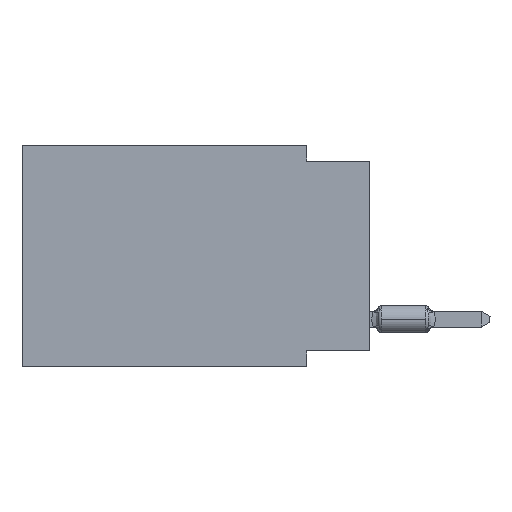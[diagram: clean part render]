
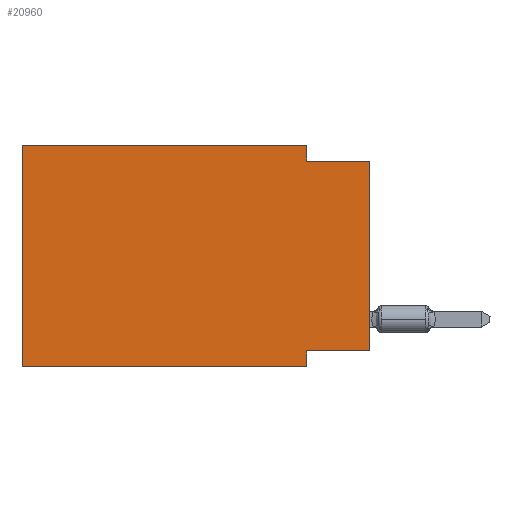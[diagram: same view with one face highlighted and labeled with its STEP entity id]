
A CAD part, left-side view. The second image highlights one B-rep face of the part: STEP entity #20960.
In plain terms, the highlighted planar face has unit normal (-1, 0, 0).
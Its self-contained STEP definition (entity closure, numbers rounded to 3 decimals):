
#476 = FACE_OUTER_BOUND ( 'NONE', #23184, .T. ) ;
#576 = VECTOR ( 'NONE', #2440, 1000. ) ;
#754 = VECTOR ( 'NONE', #22499, 1000. ) ;
#2308 = VECTOR ( 'NONE', #8924, 1000. ) ;
#2319 = CARTESIAN_POINT ( 'NONE',  ( 0., 0., -8.255 ) ) ;
#2440 = DIRECTION ( 'NONE',  ( 0., -1., 0. ) ) ;
#2577 = CARTESIAN_POINT ( 'NONE',  ( 0., 13.97, -8.89 ) ) ;
#3398 = CARTESIAN_POINT ( 'NONE',  ( 0., 13.97, 0. ) ) ;
#3448 = CARTESIAN_POINT ( 'NONE',  ( 0., 0., 0. ) ) ;
#4347 = LINE ( 'NONE', #23652, #9080 ) ;
#4489 = DIRECTION ( 'NONE',  ( 0., 0., -1. ) ) ;
#5079 = LINE ( 'NONE', #9390, #754 ) ;
#5644 = EDGE_CURVE ( 'NONE', #26869, #13309, #14357, .T. ) ;
#6349 = LINE ( 'NONE', #25778, #28345 ) ;
#6701 = VECTOR ( 'NONE', #14456, 1000. ) ;
#6781 = CARTESIAN_POINT ( 'NONE',  ( 0., 13.97, 0. ) ) ;
#8314 = EDGE_CURVE ( 'NONE', #26125, #23424, #24311, .T. ) ;
#8924 = DIRECTION ( 'NONE',  ( 0., 1., 0. ) ) ;
#9080 = VECTOR ( 'NONE', #4489, 1000. ) ;
#9188 = VECTOR ( 'NONE', #10026, 1000. ) ;
#9364 = PLANE ( 'NONE',  #10149 ) ;
#9390 = CARTESIAN_POINT ( 'NONE',  ( 0., 13.97, 0. ) ) ;
#9505 = ORIENTED_EDGE ( 'NONE', *, *, #5644, .F. ) ;
#9568 = LINE ( 'NONE', #2319, #2308 ) ;
#10026 = DIRECTION ( 'NONE',  ( 0., -1., 0. ) ) ;
#10149 = AXIS2_PLACEMENT_3D ( 'NONE', #6781, #24338, #18153 ) ;
#10439 = ORIENTED_EDGE ( 'NONE', *, *, #8314, .T. ) ;
#10589 = VECTOR ( 'NONE', #23037, 1000. ) ;
#10621 = VERTEX_POINT ( 'NONE', #19790 ) ;
#11587 = ORIENTED_EDGE ( 'NONE', *, *, #17663, .F. ) ;
#11847 = CARTESIAN_POINT ( 'NONE',  ( 0., 2.54, -0.635 ) ) ;
#13309 = VERTEX_POINT ( 'NONE', #15244 ) ;
#14181 = CARTESIAN_POINT ( 'NONE',  ( 0., 2.54, 0. ) ) ;
#14354 = ORIENTED_EDGE ( 'NONE', *, *, #15522, .F. ) ;
#14357 = LINE ( 'NONE', #3398, #9188 ) ;
#14456 = DIRECTION ( 'NONE',  ( 0., 0., -1. ) ) ;
#14462 = VERTEX_POINT ( 'NONE', #11847 ) ;
#14656 = EDGE_CURVE ( 'NONE', #14462, #28350, #6349, .T. ) ;
#15186 = ORIENTED_EDGE ( 'NONE', *, *, #15302, .F. ) ;
#15244 = CARTESIAN_POINT ( 'NONE',  ( 0., 2.54, 0. ) ) ;
#15302 = EDGE_CURVE ( 'NONE', #13309, #14462, #25393, .T. ) ;
#15522 = EDGE_CURVE ( 'NONE', #26125, #26869, #5079, .T. ) ;
#16897 = CARTESIAN_POINT ( 'NONE',  ( 0., 13.97, 0. ) ) ;
#17663 = EDGE_CURVE ( 'NONE', #21142, #23424, #4347, .T. ) ;
#18068 = CARTESIAN_POINT ( 'NONE',  ( 0., 0., -0.635 ) ) ;
#18153 = DIRECTION ( 'NONE',  ( 0., 0., -1. ) ) ;
#18716 = CARTESIAN_POINT ( 'NONE',  ( 0., 2.54, -8.255 ) ) ;
#19790 = CARTESIAN_POINT ( 'NONE',  ( 0., 0., -8.255 ) ) ;
#20401 = EDGE_CURVE ( 'NONE', #10621, #21142, #9568, .T. ) ;
#20755 = CARTESIAN_POINT ( 'NONE',  ( 0., 13.97, -8.89 ) ) ;
#20960 = ADVANCED_FACE ( 'NONE', ( #476 ), #9364, .F. ) ;
#21142 = VERTEX_POINT ( 'NONE', #18716 ) ;
#22234 = EDGE_CURVE ( 'NONE', #10621, #28350, #23180, .T. ) ;
#22375 = CARTESIAN_POINT ( 'NONE',  ( 0., 2.54, -8.89 ) ) ;
#22499 = DIRECTION ( 'NONE',  ( 0., 0., 1. ) ) ;
#22644 = ORIENTED_EDGE ( 'NONE', *, *, #22234, .T. ) ;
#23037 = DIRECTION ( 'NONE',  ( 0., 0., 1. ) ) ;
#23180 = LINE ( 'NONE', #3448, #10589 ) ;
#23184 = EDGE_LOOP ( 'NONE', ( #22644, #24193, #15186, #9505, #14354, #10439, #11587, #24804 ) ) ;
#23424 = VERTEX_POINT ( 'NONE', #22375 ) ;
#23652 = CARTESIAN_POINT ( 'NONE',  ( 0., 2.54, -8.89 ) ) ;
#23911 = DIRECTION ( 'NONE',  ( 0., -1., 0. ) ) ;
#24193 = ORIENTED_EDGE ( 'NONE', *, *, #14656, .F. ) ;
#24311 = LINE ( 'NONE', #2577, #576 ) ;
#24338 = DIRECTION ( 'NONE',  ( 1., 0., 0. ) ) ;
#24804 = ORIENTED_EDGE ( 'NONE', *, *, #20401, .F. ) ;
#25393 = LINE ( 'NONE', #14181, #6701 ) ;
#25778 = CARTESIAN_POINT ( 'NONE',  ( 0., 0., -0.635 ) ) ;
#26125 = VERTEX_POINT ( 'NONE', #20755 ) ;
#26869 = VERTEX_POINT ( 'NONE', #16897 ) ;
#28345 = VECTOR ( 'NONE', #23911, 1000. ) ;
#28350 = VERTEX_POINT ( 'NONE', #18068 ) ;
